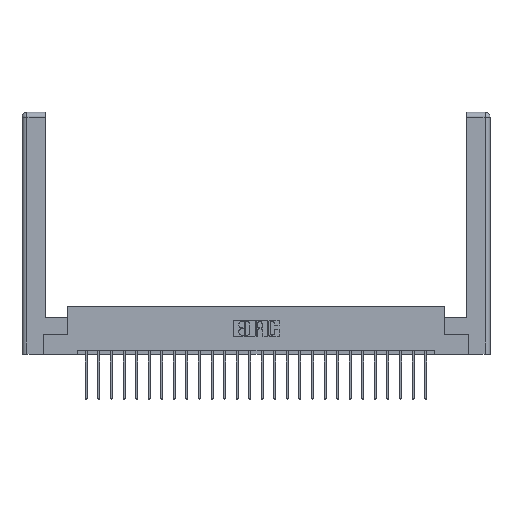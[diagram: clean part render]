
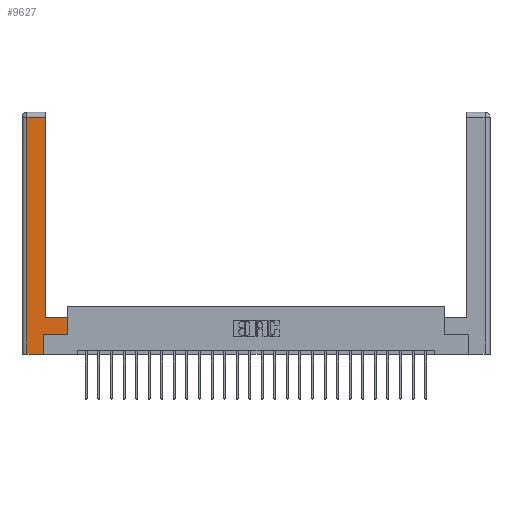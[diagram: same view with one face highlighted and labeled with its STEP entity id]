
A CAD part, top view. The second image highlights one B-rep face of the part: STEP entity #9627.
In plain terms, the highlighted planar face has unit normal (0, 0, 1).
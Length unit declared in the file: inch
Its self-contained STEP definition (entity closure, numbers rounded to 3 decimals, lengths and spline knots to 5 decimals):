
#287 = DIRECTION ( 'NONE',  ( 1., 0., 0. ) ) ;
#511 = VERTEX_POINT ( 'NONE', #11291 ) ;
#668 = EDGE_CURVE ( 'NONE', #5644, #23714, #16561, .T. ) ;
#740 = VECTOR ( 'NONE', #287, 39.37008 ) ;
#1078 = EDGE_CURVE ( 'NONE', #18067, #23654, #16537, .T. ) ;
#1293 = ORIENTED_EDGE ( 'NONE', *, *, #1078, .T. ) ;
#1403 = EDGE_CURVE ( 'NONE', #22252, #5644, #8932, .T. ) ;
#2575 = VERTEX_POINT ( 'NONE', #17558 ) ;
#2756 = AXIS2_PLACEMENT_3D ( 'NONE', #6460, #20583, #4612 ) ;
#4612 = DIRECTION ( 'NONE',  ( -1., 0., 0. ) ) ;
#5396 = CARTESIAN_POINT ( 'NONE',  ( 0.0615, 2.94, 0. ) ) ;
#5644 = VERTEX_POINT ( 'NONE', #11421 ) ;
#6460 = CARTESIAN_POINT ( 'NONE',  ( 0., 0., 0. ) ) ;
#6873 = EDGE_CURVE ( 'NONE', #511, #2575, #22199, .T. ) ;
#6876 = DIRECTION ( 'NONE',  ( 1., 0., 0. ) ) ;
#7104 = CARTESIAN_POINT ( 'NONE',  ( 0.0615, 0., 0. ) ) ;
#8272 = VERTEX_POINT ( 'NONE', #5396 ) ;
#8350 = VECTOR ( 'NONE', #19068, 39.37008 ) ;
#8632 = VECTOR ( 'NONE', #23672, 39.37008 ) ;
#8932 = LINE ( 'NONE', #16432, #740 ) ;
#8972 = CARTESIAN_POINT ( 'NONE',  ( 0.265, 0., 0. ) ) ;
#9137 = LINE ( 'NONE', #20058, #16712 ) ;
#9206 = DIRECTION ( 'NONE',  ( -1., 0., 0. ) ) ;
#9627 = ADVANCED_FACE ( 'NONE', ( #21133 ), #18548, .F. ) ;
#11291 = CARTESIAN_POINT ( 'NONE',  ( 0.0615, 0., 0. ) ) ;
#11421 = CARTESIAN_POINT ( 'NONE',  ( 0.565, 0.245, 0. ) ) ;
#11819 = ORIENTED_EDGE ( 'NONE', *, *, #24147, .T. ) ;
#12827 = ORIENTED_EDGE ( 'NONE', *, *, #6873, .T. ) ;
#13285 = DIRECTION ( 'NONE',  ( 0., -1., 0. ) ) ;
#13738 = CARTESIAN_POINT ( 'NONE',  ( 0.295, 3., 0. ) ) ;
#13923 = ORIENTED_EDGE ( 'NONE', *, *, #25885, .T. ) ;
#14357 = VECTOR ( 'NONE', #17021, 39.37008 ) ;
#14833 = LINE ( 'NONE', #21147, #19586 ) ;
#15054 = ORIENTED_EDGE ( 'NONE', *, *, #24152, .T. ) ;
#15103 = ORIENTED_EDGE ( 'NONE', *, *, #668, .T. ) ;
#15950 = CARTESIAN_POINT ( 'NONE',  ( 0.295, 2.94, 0. ) ) ;
#16432 = CARTESIAN_POINT ( 'NONE',  ( 0.565, 0.245, 0. ) ) ;
#16537 = LINE ( 'NONE', #13738, #8632 ) ;
#16561 = LINE ( 'NONE', #25284, #8350 ) ;
#16639 = ORIENTED_EDGE ( 'NONE', *, *, #1403, .T. ) ;
#16712 = VECTOR ( 'NONE', #17938, 39.37008 ) ;
#17021 = DIRECTION ( 'NONE',  ( -1., 0., 0. ) ) ;
#17066 = CARTESIAN_POINT ( 'NONE',  ( 0.265, 0.245, 0. ) ) ;
#17558 = CARTESIAN_POINT ( 'NONE',  ( 0.265, 0., 0. ) ) ;
#17938 = DIRECTION ( 'NONE',  ( 0., 1., 0. ) ) ;
#18067 = VERTEX_POINT ( 'NONE', #24382 ) ;
#18163 = LINE ( 'NONE', #25096, #14357 ) ;
#18548 = PLANE ( 'NONE',  #2756 ) ;
#19068 = DIRECTION ( 'NONE',  ( 0., 1., 0. ) ) ;
#19586 = VECTOR ( 'NONE', #9206, 39.37008 ) ;
#20058 = CARTESIAN_POINT ( 'NONE',  ( 0.265, 0.245, 0. ) ) ;
#20583 = DIRECTION ( 'NONE',  ( 0., 0., -1. ) ) ;
#21133 = FACE_OUTER_BOUND ( 'NONE', #24011, .T. ) ;
#21147 = CARTESIAN_POINT ( 'NONE',  ( 0.295, 0.45, 0. ) ) ;
#22140 = LINE ( 'NONE', #7104, #22436 ) ;
#22199 = LINE ( 'NONE', #8972, #25401 ) ;
#22252 = VERTEX_POINT ( 'NONE', #17066 ) ;
#22436 = VECTOR ( 'NONE', #13285, 39.37008 ) ;
#23654 = VERTEX_POINT ( 'NONE', #15950 ) ;
#23672 = DIRECTION ( 'NONE',  ( 0., 1., 0. ) ) ;
#23714 = VERTEX_POINT ( 'NONE', #23771 ) ;
#23771 = CARTESIAN_POINT ( 'NONE',  ( 0.565, 0.45, 0. ) ) ;
#24011 = EDGE_LOOP ( 'NONE', ( #1293, #13923, #15054, #12827, #24267, #16639, #15103, #11819 ) ) ;
#24147 = EDGE_CURVE ( 'NONE', #23714, #18067, #14833, .T. ) ;
#24152 = EDGE_CURVE ( 'NONE', #8272, #511, #22140, .T. ) ;
#24267 = ORIENTED_EDGE ( 'NONE', *, *, #24437, .T. ) ;
#24382 = CARTESIAN_POINT ( 'NONE',  ( 0.295, 0.45, 0. ) ) ;
#24437 = EDGE_CURVE ( 'NONE', #2575, #22252, #9137, .T. ) ;
#25096 = CARTESIAN_POINT ( 'NONE',  ( 0.0615, 2.94, 0. ) ) ;
#25284 = CARTESIAN_POINT ( 'NONE',  ( 0.565, 0.45, 0. ) ) ;
#25401 = VECTOR ( 'NONE', #6876, 39.37008 ) ;
#25885 = EDGE_CURVE ( 'NONE', #23654, #8272, #18163, .T. ) ;
